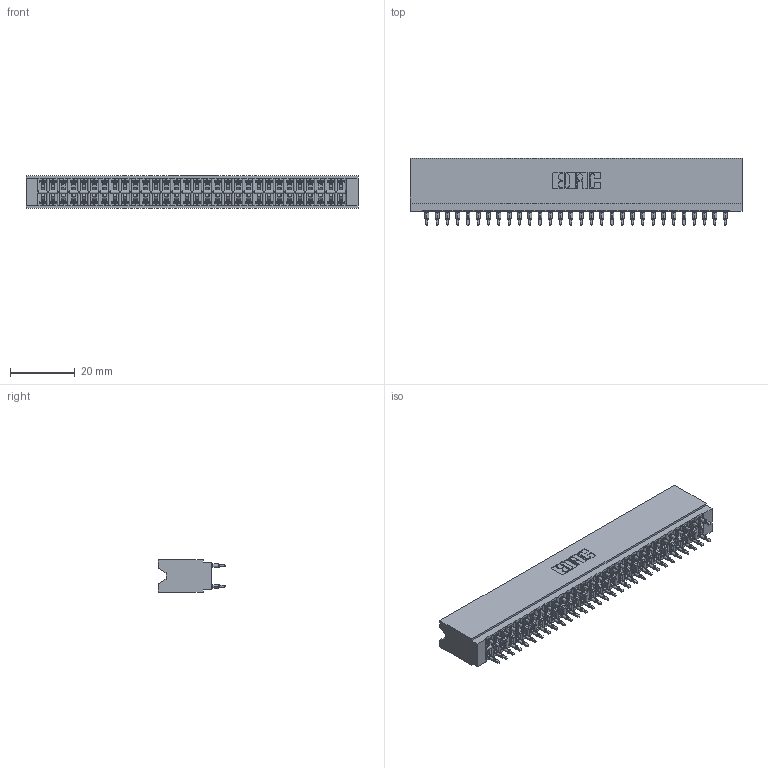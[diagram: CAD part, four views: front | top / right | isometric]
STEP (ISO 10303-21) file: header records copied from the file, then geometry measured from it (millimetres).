
FILE_DESCRIPTION (( 'STEP AP203' ), '1' );
FILE_NAME ('746-060-560-206.STEP', '2026-02-27T20:36:31', ( '' ), ( '' ), 'SwSTEP 2.0', 'SolidWorks 2023', '' );
FILE_SCHEMA (( 'CONFIG_CONTROL_DESIGN' ));
Length unit declared in the file: millimetre
Products named in the file (3): 746-292-001_560; 746-060-560-206; 746 Part_.515 Slot Depth - 06
Assembly tree (61 placements, depth 2):
  746-060-560-206
    746 Part_.515 Slot Depth - 06
    746-292-001_560  x60
Bounding box: 102.49 x 20.82 x 9.91 mm (x, y, z)
Volume: 11247.9 mm3; surface area: 18817.1 mm2
Topology: 61 solids, 61 shells, 5768 faces, 16045 edges, 10285 vertices
Faces by surface type: plane 2876, cylinder 1332, bspline 1200, torus 360
Entity records: 48196 total; most frequent: CARTESIAN_POINT 9682, ORIENTED_EDGE 8254, DIRECTION 6919, EDGE_CURVE 4127, VECTOR 3635, LINE 3635, VERTEX_POINT 2733, AXIS2_PLACEMENT_3D 1642
